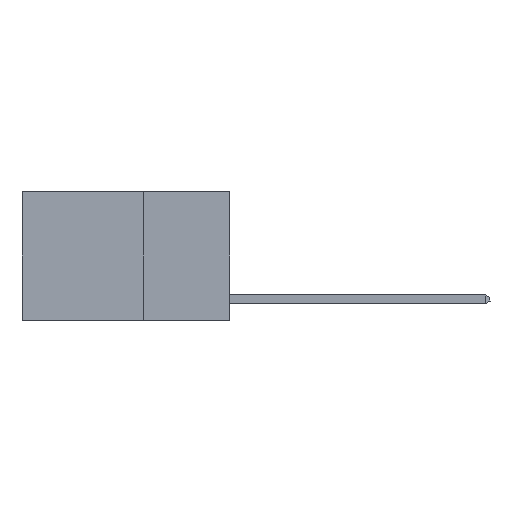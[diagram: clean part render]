
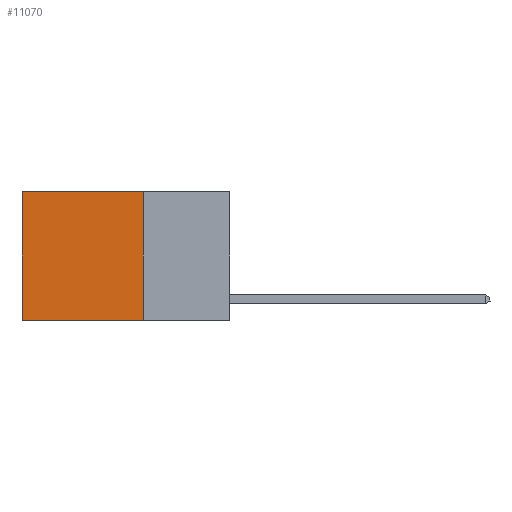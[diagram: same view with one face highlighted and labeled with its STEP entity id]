
A CAD part, left-side view. The second image highlights one B-rep face of the part: STEP entity #11070.
In plain terms, the highlighted planar face has unit normal (-1, 0, 0).
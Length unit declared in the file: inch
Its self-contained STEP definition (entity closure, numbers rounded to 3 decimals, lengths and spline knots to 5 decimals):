
#373 = AXIS2_PLACEMENT_3D ( 'NONE', #13390, #9673, #6237 ) ;
#471 = CARTESIAN_POINT ( 'NONE',  ( 0.2625, 0.25, 0. ) ) ;
#1317 = VECTOR ( 'NONE', #4555, 39.37008 ) ;
#3109 = EDGE_CURVE ( 'NONE', #8153, #12477, #14541, .T. ) ;
#3571 = EDGE_CURVE ( 'NONE', #8153, #8926, #12754, .T. ) ;
#4555 = DIRECTION ( 'NONE',  ( 0., 0., -1. ) ) ;
#4629 = CARTESIAN_POINT ( 'NONE',  ( 0.2625, 0.6, 0. ) ) ;
#4810 = CARTESIAN_POINT ( 'NONE',  ( 0.2625, 0.25, 0. ) ) ;
#5217 = VERTEX_POINT ( 'NONE', #12480 ) ;
#6237 = DIRECTION ( 'NONE',  ( 0., 0., -1. ) ) ;
#6418 = DIRECTION ( 'NONE',  ( 0., 1., 0. ) ) ;
#6726 = LINE ( 'NONE', #4629, #1317 ) ;
#7167 = VECTOR ( 'NONE', #6418, 39.37008 ) ;
#7467 = CARTESIAN_POINT ( 'NONE',  ( 0.2625, 0.25, -0.37 ) ) ;
#7524 = FACE_OUTER_BOUND ( 'NONE', #11466, .T. ) ;
#8153 = VERTEX_POINT ( 'NONE', #471 ) ;
#8231 = ORIENTED_EDGE ( 'NONE', *, *, #3571, .F. ) ;
#8245 = ORIENTED_EDGE ( 'NONE', *, *, #10369, .T. ) ;
#8535 = VECTOR ( 'NONE', #10995, 39.37008 ) ;
#8926 = VERTEX_POINT ( 'NONE', #13700 ) ;
#9673 = DIRECTION ( 'NONE',  ( 1., 0., 0. ) ) ;
#9899 = PLANE ( 'NONE',  #373 ) ;
#10369 = EDGE_CURVE ( 'NONE', #12477, #5217, #6726, .T. ) ;
#10995 = DIRECTION ( 'NONE',  ( 0., 1., 0. ) ) ;
#11070 = ADVANCED_FACE ( 'NONE', ( #7524 ), #9899, .F. ) ;
#11466 = EDGE_LOOP ( 'NONE', ( #8245, #13077, #8231, #13468 ) ) ;
#12477 = VERTEX_POINT ( 'NONE', #14814 ) ;
#12480 = CARTESIAN_POINT ( 'NONE',  ( 0.2625, 0.6, -0.37 ) ) ;
#12491 = CARTESIAN_POINT ( 'NONE',  ( 0.2625, 0.25, 0. ) ) ;
#12754 = LINE ( 'NONE', #4810, #14645 ) ;
#13077 = ORIENTED_EDGE ( 'NONE', *, *, #14514, .F. ) ;
#13194 = LINE ( 'NONE', #7467, #7167 ) ;
#13390 = CARTESIAN_POINT ( 'NONE',  ( 0.2625, 0.25, 0. ) ) ;
#13468 = ORIENTED_EDGE ( 'NONE', *, *, #3109, .T. ) ;
#13700 = CARTESIAN_POINT ( 'NONE',  ( 0.2625, 0.25, -0.37 ) ) ;
#14020 = DIRECTION ( 'NONE',  ( 0., 0., -1. ) ) ;
#14514 = EDGE_CURVE ( 'NONE', #8926, #5217, #13194, .T. ) ;
#14541 = LINE ( 'NONE', #12491, #8535 ) ;
#14645 = VECTOR ( 'NONE', #14020, 39.37008 ) ;
#14814 = CARTESIAN_POINT ( 'NONE',  ( 0.2625, 0.6, 0. ) ) ;
